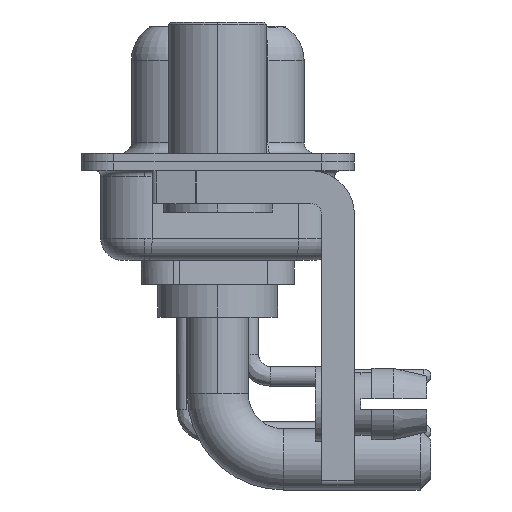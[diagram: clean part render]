
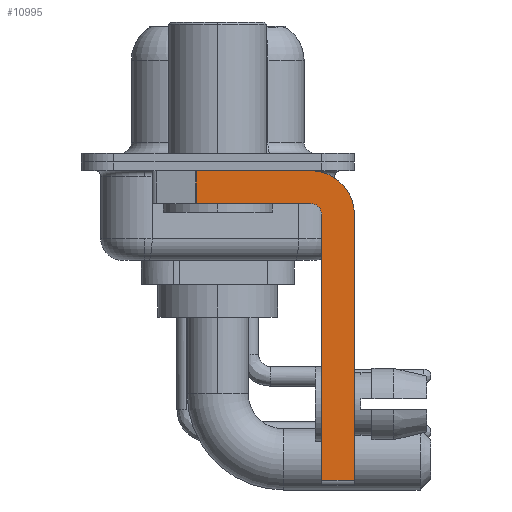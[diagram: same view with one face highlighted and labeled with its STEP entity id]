
A CAD part, left-side view. The second image highlights one B-rep face of the part: STEP entity #10995.
In plain terms, the highlighted planar face has unit normal (-1, 0, 0).
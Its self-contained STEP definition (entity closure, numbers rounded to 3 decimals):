
#775 = ORIENTED_EDGE ( 'NONE', *, *, #25303, .T. ) ;
#908 = AXIS2_PLACEMENT_3D ( 'NONE', #1512, #17786, #9598 ) ;
#1166 = EDGE_CURVE ( 'NONE', #6429, #13918, #8113, .T. ) ;
#1503 = LINE ( 'NONE', #23616, #14219 ) ;
#1512 = CARTESIAN_POINT ( 'NONE',  ( -2.9, -4.25, -2.4 ) ) ;
#1811 = CARTESIAN_POINT ( 'NONE',  ( -2.9, -6.25, -14.55 ) ) ;
#2150 = VERTEX_POINT ( 'NONE', #4411 ) ;
#2416 = EDGE_LOOP ( 'NONE', ( #22665, #4535, #21645, #5684, #15153, #775, #10220, #2898 ) ) ;
#2672 = VERTEX_POINT ( 'NONE', #1811 ) ;
#2898 = ORIENTED_EDGE ( 'NONE', *, *, #1166, .F. ) ;
#2970 = DIRECTION ( 'NONE',  ( 0., 0., -1. ) ) ;
#3306 = VECTOR ( 'NONE', #5546, 1000. ) ;
#3911 = VERTEX_POINT ( 'NONE', #12987 ) ;
#4411 = CARTESIAN_POINT ( 'NONE',  ( -2.9, 0.978, -1.9 ) ) ;
#4535 = ORIENTED_EDGE ( 'NONE', *, *, #10229, .T. ) ;
#5546 = DIRECTION ( 'NONE',  ( 0., 1., 0. ) ) ;
#5684 = ORIENTED_EDGE ( 'NONE', *, *, #8192, .F. ) ;
#5862 = VERTEX_POINT ( 'NONE', #18914 ) ;
#6429 = VERTEX_POINT ( 'NONE', #10805 ) ;
#6440 = CARTESIAN_POINT ( 'NONE',  ( -2.9, -4.75, -2.4 ) ) ;
#6459 = VERTEX_POINT ( 'NONE', #6440 ) ;
#6615 = CARTESIAN_POINT ( 'NONE',  ( -2.9, -4.25, -2.4 ) ) ;
#7001 = VERTEX_POINT ( 'NONE', #26007 ) ;
#7004 = EDGE_CURVE ( 'NONE', #5862, #6429, #9999, .T. ) ;
#7278 = DIRECTION ( 'NONE',  ( 0., -1., 0. ) ) ;
#7401 = CARTESIAN_POINT ( 'NONE',  ( -2.9, -4.25, -1.9 ) ) ;
#7664 = DIRECTION ( 'NONE',  ( 0., 0., -1. ) ) ;
#8113 = CIRCLE ( 'NONE', #908, 2. ) ;
#8192 = EDGE_CURVE ( 'NONE', #6459, #7001, #25528, .T. ) ;
#8329 = DIRECTION ( 'NONE',  ( -1., 0., 0. ) ) ;
#8563 = VECTOR ( 'NONE', #15035, 1000. ) ;
#8820 = CARTESIAN_POINT ( 'NONE',  ( -2.9, -6.25, -2.4 ) ) ;
#8873 = CARTESIAN_POINT ( 'NONE',  ( -2.9, -4.25, -14.55 ) ) ;
#8935 = LINE ( 'NONE', #14905, #8563 ) ;
#9598 = DIRECTION ( 'NONE',  ( 0., 0., -1. ) ) ;
#9999 = LINE ( 'NONE', #18059, #12830 ) ;
#10220 = ORIENTED_EDGE ( 'NONE', *, *, #17864, .F. ) ;
#10229 = EDGE_CURVE ( 'NONE', #5862, #2150, #1503, .T. ) ;
#10690 = DIRECTION ( 'NONE',  ( 0., 0., -1. ) ) ;
#10805 = CARTESIAN_POINT ( 'NONE',  ( -2.9, -4.25, -0.4 ) ) ;
#10995 = ADVANCED_FACE ( 'NONE', ( #11070 ), #14789, .F. ) ;
#11070 = FACE_OUTER_BOUND ( 'NONE', #2416, .T. ) ;
#12830 = VECTOR ( 'NONE', #16333, 1000. ) ;
#12987 = CARTESIAN_POINT ( 'NONE',  ( -2.9, -4.75, -14.55 ) ) ;
#13918 = VERTEX_POINT ( 'NONE', #8820 ) ;
#14122 = AXIS2_PLACEMENT_3D ( 'NONE', #6615, #8329, #22506 ) ;
#14219 = VECTOR ( 'NONE', #2970, 1000. ) ;
#14789 = PLANE ( 'NONE',  #17631 ) ;
#14905 = CARTESIAN_POINT ( 'NONE',  ( -2.9, -4.75, -14.8 ) ) ;
#15035 = DIRECTION ( 'NONE',  ( 0., 0., 1. ) ) ;
#15153 = ORIENTED_EDGE ( 'NONE', *, *, #21921, .F. ) ;
#15617 = LINE ( 'NONE', #23699, #18987 ) ;
#16333 = DIRECTION ( 'NONE',  ( 0., -1., 0. ) ) ;
#16549 = EDGE_CURVE ( 'NONE', #7001, #2150, #23694, .T. ) ;
#17210 = LINE ( 'NONE', #8873, #25093 ) ;
#17631 = AXIS2_PLACEMENT_3D ( 'NONE', #20888, #20751, #10690 ) ;
#17786 = DIRECTION ( 'NONE',  ( 1., 0., 0. ) ) ;
#17864 = EDGE_CURVE ( 'NONE', #13918, #2672, #15617, .T. ) ;
#18059 = CARTESIAN_POINT ( 'NONE',  ( -2.9, 3., -0.4 ) ) ;
#18914 = CARTESIAN_POINT ( 'NONE',  ( -2.9, 0.978, -0.4 ) ) ;
#18987 = VECTOR ( 'NONE', #7664, 1000. ) ;
#20751 = DIRECTION ( 'NONE',  ( 1., 0., 0. ) ) ;
#20888 = CARTESIAN_POINT ( 'NONE',  ( -2.9, -4.25, -2.4 ) ) ;
#21645 = ORIENTED_EDGE ( 'NONE', *, *, #16549, .F. ) ;
#21921 = EDGE_CURVE ( 'NONE', #3911, #6459, #8935, .T. ) ;
#22506 = DIRECTION ( 'NONE',  ( 0., 0., 1. ) ) ;
#22665 = ORIENTED_EDGE ( 'NONE', *, *, #7004, .F. ) ;
#23616 = CARTESIAN_POINT ( 'NONE',  ( -2.9, 0.978, -1.9 ) ) ;
#23694 = LINE ( 'NONE', #7401, #3306 ) ;
#23699 = CARTESIAN_POINT ( 'NONE',  ( -2.9, -6.25, -2.4 ) ) ;
#25093 = VECTOR ( 'NONE', #7278, 1000. ) ;
#25303 = EDGE_CURVE ( 'NONE', #3911, #2672, #17210, .T. ) ;
#25528 = CIRCLE ( 'NONE', #14122, 0.5 ) ;
#26007 = CARTESIAN_POINT ( 'NONE',  ( -2.9, -4.25, -1.9 ) ) ;
